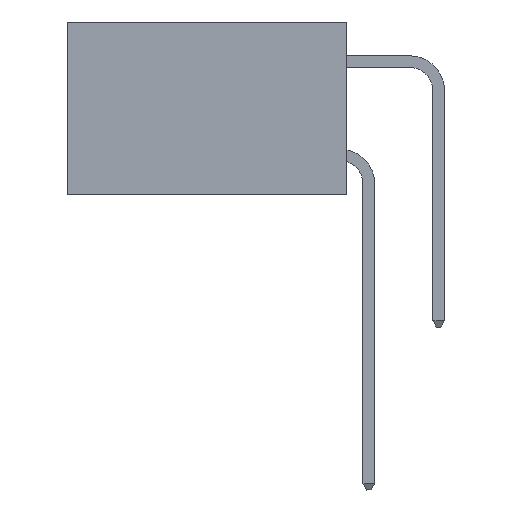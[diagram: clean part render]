
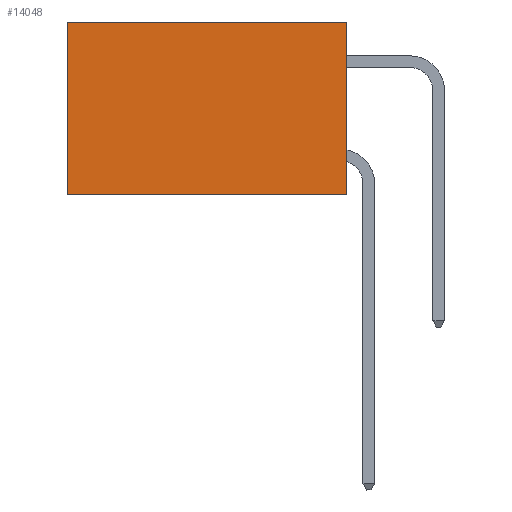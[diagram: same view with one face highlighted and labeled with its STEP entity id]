
A CAD part, left-side view. The second image highlights one B-rep face of the part: STEP entity #14048.
In plain terms, the highlighted planar face has unit normal (-1, 0, 0).
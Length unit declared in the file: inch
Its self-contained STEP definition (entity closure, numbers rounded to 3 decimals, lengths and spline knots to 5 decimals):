
#489 = CARTESIAN_POINT ( 'NONE',  ( 0.2875, 0., 0. ) ) ;
#1638 = DIRECTION ( 'NONE',  ( 0., 0., -1. ) ) ;
#2807 = EDGE_CURVE ( 'NONE', #20898, #17289, #6660, .T. ) ;
#3592 = VECTOR ( 'NONE', #4056, 39.37008 ) ;
#4056 = DIRECTION ( 'NONE',  ( 0., 1., 0. ) ) ;
#4778 = DIRECTION ( 'NONE',  ( 0., 0., -1. ) ) ;
#4988 = ORIENTED_EDGE ( 'NONE', *, *, #2807, .F. ) ;
#5244 = ORIENTED_EDGE ( 'NONE', *, *, #7746, .F. ) ;
#5441 = VECTOR ( 'NONE', #1638, 39.37008 ) ;
#5593 = LINE ( 'NONE', #15123, #6453 ) ;
#5966 = DIRECTION ( 'NONE',  ( 0., 0., -1. ) ) ;
#6035 = CARTESIAN_POINT ( 'NONE',  ( 0.2875, 0., -0.37 ) ) ;
#6453 = VECTOR ( 'NONE', #4778, 39.37008 ) ;
#6660 = LINE ( 'NONE', #18050, #3592 ) ;
#7302 = FACE_OUTER_BOUND ( 'NONE', #10564, .T. ) ;
#7500 = VERTEX_POINT ( 'NONE', #14419 ) ;
#7746 = EDGE_CURVE ( 'NONE', #7500, #20898, #5593, .T. ) ;
#8469 = CARTESIAN_POINT ( 'NONE',  ( 0.2875, 0.6, 0. ) ) ;
#9198 = EDGE_CURVE ( 'NONE', #7500, #9290, #17682, .T. ) ;
#9290 = VERTEX_POINT ( 'NONE', #14736 ) ;
#10564 = EDGE_LOOP ( 'NONE', ( #21063, #4988, #5244, #22419 ) ) ;
#11363 = VECTOR ( 'NONE', #18216, 39.37008 ) ;
#12713 = EDGE_CURVE ( 'NONE', #9290, #17289, #19430, .T. ) ;
#13518 = DIRECTION ( 'NONE',  ( 1., 0., 0. ) ) ;
#14048 = ADVANCED_FACE ( 'NONE', ( #7302 ), #14396, .F. ) ;
#14396 = PLANE ( 'NONE',  #18195 ) ;
#14419 = CARTESIAN_POINT ( 'NONE',  ( 0.2875, 0., 0. ) ) ;
#14594 = CARTESIAN_POINT ( 'NONE',  ( 0.2875, 0.6, -0.37 ) ) ;
#14736 = CARTESIAN_POINT ( 'NONE',  ( 0.2875, 0.6, 0. ) ) ;
#15123 = CARTESIAN_POINT ( 'NONE',  ( 0.2875, 0., 0. ) ) ;
#15709 = CARTESIAN_POINT ( 'NONE',  ( 0.2875, 0., 0. ) ) ;
#17289 = VERTEX_POINT ( 'NONE', #14594 ) ;
#17682 = LINE ( 'NONE', #489, #11363 ) ;
#18050 = CARTESIAN_POINT ( 'NONE',  ( 0.2875, 0., -0.37 ) ) ;
#18195 = AXIS2_PLACEMENT_3D ( 'NONE', #15709, #13518, #5966 ) ;
#18216 = DIRECTION ( 'NONE',  ( 0., 1., 0. ) ) ;
#19430 = LINE ( 'NONE', #8469, #5441 ) ;
#20898 = VERTEX_POINT ( 'NONE', #6035 ) ;
#21063 = ORIENTED_EDGE ( 'NONE', *, *, #12713, .T. ) ;
#22419 = ORIENTED_EDGE ( 'NONE', *, *, #9198, .T. ) ;
